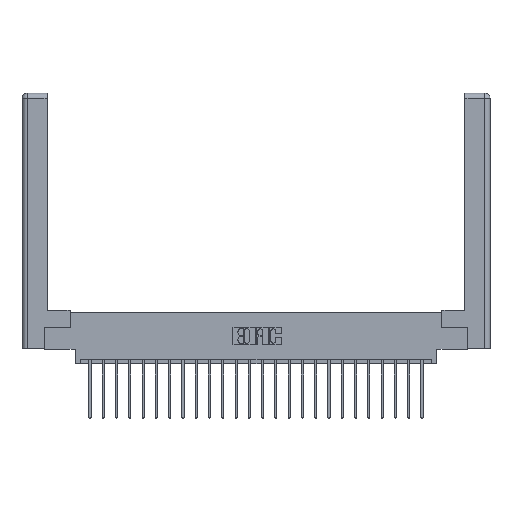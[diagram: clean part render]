
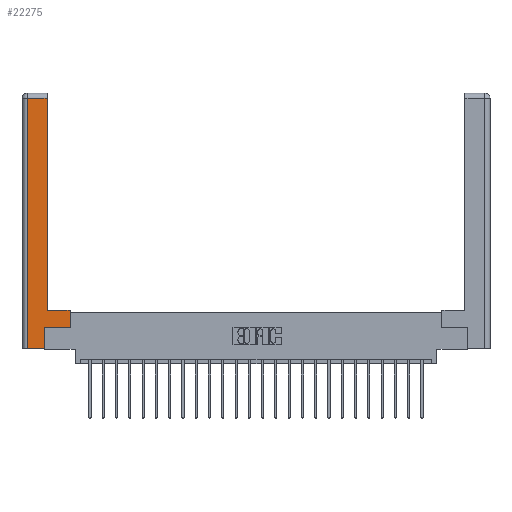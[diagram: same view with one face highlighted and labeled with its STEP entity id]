
A CAD part, top view. The second image highlights one B-rep face of the part: STEP entity #22275.
In plain terms, the highlighted planar face has unit normal (0, 0, 1).
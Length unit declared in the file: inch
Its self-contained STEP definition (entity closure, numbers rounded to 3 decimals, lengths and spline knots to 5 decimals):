
#139 = VECTOR ( 'NONE', #21801, 39.37008 ) ;
#150 = CARTESIAN_POINT ( 'NONE',  ( 0.295, 0.45, 0. ) ) ;
#729 = ORIENTED_EDGE ( 'NONE', *, *, #19765, .T. ) ;
#1349 = CARTESIAN_POINT ( 'NONE',  ( 0.265, 0.245, 0. ) ) ;
#1693 = VECTOR ( 'NONE', #5069, 39.37008 ) ;
#2098 = LINE ( 'NONE', #12509, #23845 ) ;
#2472 = CARTESIAN_POINT ( 'NONE',  ( 0.265, 0., 0. ) ) ;
#3898 = VECTOR ( 'NONE', #15978, 39.37008 ) ;
#3999 = VERTEX_POINT ( 'NONE', #18394 ) ;
#5069 = DIRECTION ( 'NONE',  ( 0., 1., 0. ) ) ;
#5810 = CARTESIAN_POINT ( 'NONE',  ( 0.565, 0.45, 0. ) ) ;
#5864 = VERTEX_POINT ( 'NONE', #18331 ) ;
#5929 = VERTEX_POINT ( 'NONE', #12342 ) ;
#6031 = VERTEX_POINT ( 'NONE', #18816 ) ;
#6646 = DIRECTION ( 'NONE',  ( 0., 1., 0. ) ) ;
#6818 = LINE ( 'NONE', #1349, #1693 ) ;
#7259 = ORIENTED_EDGE ( 'NONE', *, *, #19639, .T. ) ;
#7629 = DIRECTION ( 'NONE',  ( -1., 0., 0. ) ) ;
#9319 = LINE ( 'NONE', #2472, #3898 ) ;
#9337 = LINE ( 'NONE', #10786, #23552 ) ;
#9625 = EDGE_CURVE ( 'NONE', #23968, #5929, #9337, .T. ) ;
#10059 = VERTEX_POINT ( 'NONE', #14717 ) ;
#10064 = CARTESIAN_POINT ( 'NONE',  ( 0.295, 0.45, 0. ) ) ;
#10455 = ORIENTED_EDGE ( 'NONE', *, *, #10685, .T. ) ;
#10685 = EDGE_CURVE ( 'NONE', #5864, #12714, #22898, .T. ) ;
#10785 = AXIS2_PLACEMENT_3D ( 'NONE', #15996, #13724, #17835 ) ;
#10786 = CARTESIAN_POINT ( 'NONE',  ( 0.295, 3., 0. ) ) ;
#11113 = FACE_OUTER_BOUND ( 'NONE', #17641, .T. ) ;
#11658 = ORIENTED_EDGE ( 'NONE', *, *, #12797, .T. ) ;
#12095 = ORIENTED_EDGE ( 'NONE', *, *, #9625, .T. ) ;
#12332 = CARTESIAN_POINT ( 'NONE',  ( 0.0615, 0., 0. ) ) ;
#12342 = CARTESIAN_POINT ( 'NONE',  ( 0.295, 2.94, 0. ) ) ;
#12478 = ORIENTED_EDGE ( 'NONE', *, *, #20280, .T. ) ;
#12509 = CARTESIAN_POINT ( 'NONE',  ( 0.565, 0.245, 0. ) ) ;
#12714 = VERTEX_POINT ( 'NONE', #22351 ) ;
#12797 = EDGE_CURVE ( 'NONE', #10059, #6031, #6818, .T. ) ;
#13724 = DIRECTION ( 'NONE',  ( 0., 0., -1. ) ) ;
#14717 = CARTESIAN_POINT ( 'NONE',  ( 0.265, 0., 0. ) ) ;
#15020 = VECTOR ( 'NONE', #7629, 39.37008 ) ;
#15490 = CARTESIAN_POINT ( 'NONE',  ( 0.0615, 2.94, 0. ) ) ;
#15915 = PLANE ( 'NONE',  #10785 ) ;
#15978 = DIRECTION ( 'NONE',  ( 1., 0., 0. ) ) ;
#15996 = CARTESIAN_POINT ( 'NONE',  ( 0., 0., 0. ) ) ;
#16211 = DIRECTION ( 'NONE',  ( 0., -1., 0. ) ) ;
#16232 = LINE ( 'NONE', #15490, #15020 ) ;
#16864 = EDGE_CURVE ( 'NONE', #3999, #23968, #24942, .T. ) ;
#17641 = EDGE_LOOP ( 'NONE', ( #12095, #22334, #10455, #7259, #11658, #729, #12478, #18317 ) ) ;
#17835 = DIRECTION ( 'NONE',  ( -1., 0., 0. ) ) ;
#18237 = DIRECTION ( 'NONE',  ( 1., 0., 0. ) ) ;
#18317 = ORIENTED_EDGE ( 'NONE', *, *, #16864, .T. ) ;
#18331 = CARTESIAN_POINT ( 'NONE',  ( 0.0615, 2.94, 0. ) ) ;
#18394 = CARTESIAN_POINT ( 'NONE',  ( 0.565, 0.45, 0. ) ) ;
#18816 = CARTESIAN_POINT ( 'NONE',  ( 0.265, 0.245, 0. ) ) ;
#19639 = EDGE_CURVE ( 'NONE', #12714, #10059, #9319, .T. ) ;
#19765 = EDGE_CURVE ( 'NONE', #6031, #24527, #2098, .T. ) ;
#20280 = EDGE_CURVE ( 'NONE', #24527, #3999, #22894, .T. ) ;
#20744 = VECTOR ( 'NONE', #16211, 39.37008 ) ;
#20784 = EDGE_CURVE ( 'NONE', #5929, #5864, #16232, .T. ) ;
#21801 = DIRECTION ( 'NONE',  ( -1., 0., 0. ) ) ;
#22275 = ADVANCED_FACE ( 'NONE', ( #11113 ), #15915, .F. ) ;
#22334 = ORIENTED_EDGE ( 'NONE', *, *, #20784, .T. ) ;
#22351 = CARTESIAN_POINT ( 'NONE',  ( 0.0615, 0., 0. ) ) ;
#22894 = LINE ( 'NONE', #5810, #23508 ) ;
#22898 = LINE ( 'NONE', #12332, #20744 ) ;
#23291 = DIRECTION ( 'NONE',  ( 0., 1., 0. ) ) ;
#23508 = VECTOR ( 'NONE', #23291, 39.37008 ) ;
#23552 = VECTOR ( 'NONE', #6646, 39.37008 ) ;
#23845 = VECTOR ( 'NONE', #18237, 39.37008 ) ;
#23968 = VERTEX_POINT ( 'NONE', #150 ) ;
#24527 = VERTEX_POINT ( 'NONE', #24975 ) ;
#24942 = LINE ( 'NONE', #10064, #139 ) ;
#24975 = CARTESIAN_POINT ( 'NONE',  ( 0.565, 0.245, 0. ) ) ;
